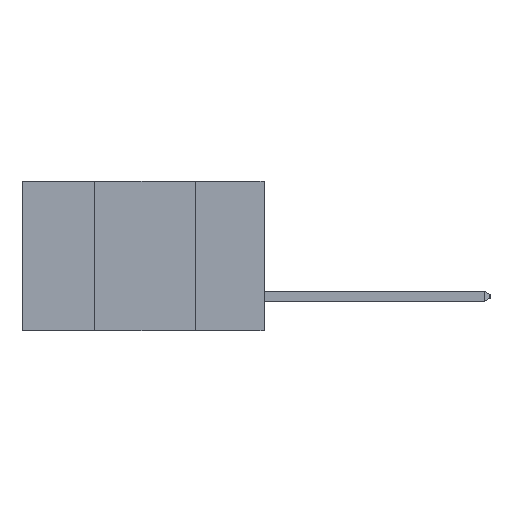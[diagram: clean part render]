
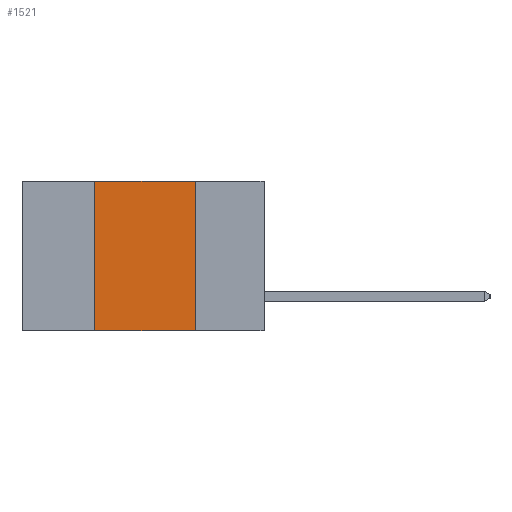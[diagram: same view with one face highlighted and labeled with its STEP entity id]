
A CAD part, left-side view. The second image highlights one B-rep face of the part: STEP entity #1521.
In plain terms, the highlighted planar face has unit normal (-1, 0, 0).
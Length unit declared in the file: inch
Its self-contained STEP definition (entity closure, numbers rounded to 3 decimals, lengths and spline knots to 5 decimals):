
#247 = VECTOR ( 'NONE', #3838, 39.37008 ) ;
#1011 = ORIENTED_EDGE ( 'NONE', *, *, #6843, .T. ) ;
#1278 = VECTOR ( 'NONE', #17485, 39.37008 ) ;
#1490 = VERTEX_POINT ( 'NONE', #14517 ) ;
#1521 = ADVANCED_FACE ( 'NONE', ( #10907 ), #10810, .F. ) ;
#1777 = CARTESIAN_POINT ( 'NONE',  ( 0., 0.17, 0. ) ) ;
#2109 = ORIENTED_EDGE ( 'NONE', *, *, #11771, .F. ) ;
#2980 = EDGE_CURVE ( 'NONE', #8524, #9535, #8625, .T. ) ;
#3514 = CARTESIAN_POINT ( 'NONE',  ( 0., 0.6, -0.37 ) ) ;
#3582 = DIRECTION ( 'NONE',  ( 0., -1., 0. ) ) ;
#3759 = DIRECTION ( 'NONE',  ( 0., 0., -1. ) ) ;
#3838 = DIRECTION ( 'NONE',  ( 0., 0., 1. ) ) ;
#4856 = AXIS2_PLACEMENT_3D ( 'NONE', #8990, #14065, #4989 ) ;
#4989 = DIRECTION ( 'NONE',  ( 0., 0., -1. ) ) ;
#6046 = CARTESIAN_POINT ( 'NONE',  ( 0., 0.17, -0.37 ) ) ;
#6843 = EDGE_CURVE ( 'NONE', #1490, #7524, #16914, .T. ) ;
#7138 = LINE ( 'NONE', #9741, #247 ) ;
#7524 = VERTEX_POINT ( 'NONE', #6046 ) ;
#8524 = VERTEX_POINT ( 'NONE', #14544 ) ;
#8625 = LINE ( 'NONE', #17431, #1278 ) ;
#8990 = CARTESIAN_POINT ( 'NONE',  ( 0., 0.6, 0. ) ) ;
#9535 = VERTEX_POINT ( 'NONE', #1777 ) ;
#9741 = CARTESIAN_POINT ( 'NONE',  ( 0., 0.42, -0.37 ) ) ;
#10810 = PLANE ( 'NONE',  #4856 ) ;
#10907 = FACE_OUTER_BOUND ( 'NONE', #18415, .T. ) ;
#11771 = EDGE_CURVE ( 'NONE', #1490, #8524, #7138, .T. ) ;
#11969 = VECTOR ( 'NONE', #3759, 39.37008 ) ;
#12515 = CARTESIAN_POINT ( 'NONE',  ( 0., 0.17, -0.37 ) ) ;
#13660 = VECTOR ( 'NONE', #3582, 39.37008 ) ;
#14065 = DIRECTION ( 'NONE',  ( 1., 0., 0. ) ) ;
#14517 = CARTESIAN_POINT ( 'NONE',  ( 0., 0.42, -0.37 ) ) ;
#14544 = CARTESIAN_POINT ( 'NONE',  ( 0., 0.42, 0. ) ) ;
#14809 = LINE ( 'NONE', #12515, #11969 ) ;
#14952 = EDGE_CURVE ( 'NONE', #9535, #7524, #14809, .T. ) ;
#15502 = ORIENTED_EDGE ( 'NONE', *, *, #2980, .F. ) ;
#16308 = ORIENTED_EDGE ( 'NONE', *, *, #14952, .F. ) ;
#16914 = LINE ( 'NONE', #3514, #13660 ) ;
#17431 = CARTESIAN_POINT ( 'NONE',  ( 0., 0.6, 0. ) ) ;
#17485 = DIRECTION ( 'NONE',  ( 0., -1., 0. ) ) ;
#18415 = EDGE_LOOP ( 'NONE', ( #16308, #15502, #2109, #1011 ) ) ;
